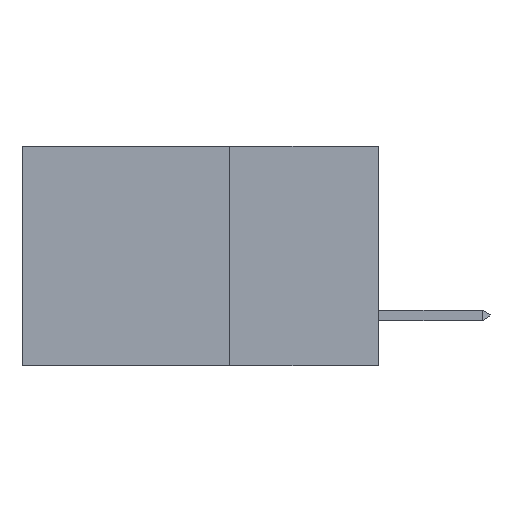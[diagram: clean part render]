
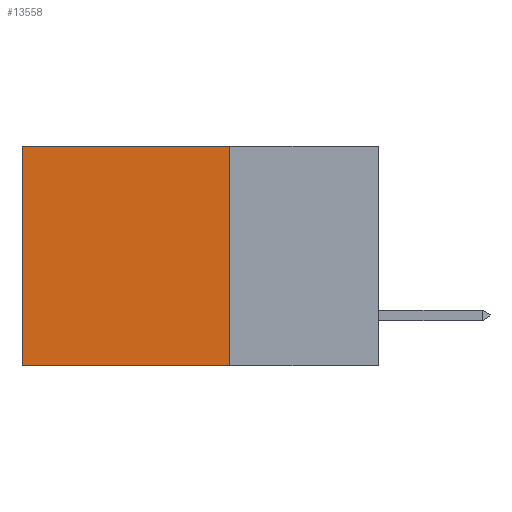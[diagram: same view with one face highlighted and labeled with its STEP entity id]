
A CAD part, left-side view. The second image highlights one B-rep face of the part: STEP entity #13558.
In plain terms, the highlighted planar face has unit normal (-1, 0, 0).
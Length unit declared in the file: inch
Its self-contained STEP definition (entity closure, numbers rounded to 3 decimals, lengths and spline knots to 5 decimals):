
#836 = ORIENTED_EDGE ( 'NONE', *, *, #20649, .T. ) ;
#1356 = CARTESIAN_POINT ( 'NONE',  ( 0.2615, 0.6, -0.37 ) ) ;
#1430 = EDGE_LOOP ( 'NONE', ( #836, #12405, #22193, #13598 ) ) ;
#1436 = DIRECTION ( 'NONE',  ( 0., 0., -1. ) ) ;
#1724 = CARTESIAN_POINT ( 'NONE',  ( 0.2615, 0.6, 0. ) ) ;
#2006 = EDGE_CURVE ( 'NONE', #5939, #5750, #13327, .T. ) ;
#3229 = DIRECTION ( 'NONE',  ( 0., 1., 0. ) ) ;
#4410 = LINE ( 'NONE', #1356, #17675 ) ;
#4940 = PLANE ( 'NONE',  #7764 ) ;
#5454 = VERTEX_POINT ( 'NONE', #18289 ) ;
#5750 = VERTEX_POINT ( 'NONE', #1724 ) ;
#5939 = VERTEX_POINT ( 'NONE', #19755 ) ;
#7031 = DIRECTION ( 'NONE',  ( 0., 1., 0. ) ) ;
#7764 = AXIS2_PLACEMENT_3D ( 'NONE', #10252, #17168, #1436 ) ;
#8415 = VECTOR ( 'NONE', #3229, 39.37008 ) ;
#8834 = CARTESIAN_POINT ( 'NONE',  ( 0.2615, 0.25, -0.37 ) ) ;
#9804 = FACE_OUTER_BOUND ( 'NONE', #1430, .T. ) ;
#10252 = CARTESIAN_POINT ( 'NONE',  ( 0.2615, 0.25, -0.37 ) ) ;
#10390 = CARTESIAN_POINT ( 'NONE',  ( 0.2615, 0.25, -0.37 ) ) ;
#12015 = LINE ( 'NONE', #8834, #19119 ) ;
#12405 = ORIENTED_EDGE ( 'NONE', *, *, #17701, .F. ) ;
#12940 = VECTOR ( 'NONE', #15413, 39.37008 ) ;
#13327 = LINE ( 'NONE', #13545, #8415 ) ;
#13545 = CARTESIAN_POINT ( 'NONE',  ( 0.2615, 0.25, 0. ) ) ;
#13558 = ADVANCED_FACE ( 'NONE', ( #9804 ), #4940, .F. ) ;
#13598 = ORIENTED_EDGE ( 'NONE', *, *, #2006, .T. ) ;
#13700 = LINE ( 'NONE', #10390, #12940 ) ;
#15413 = DIRECTION ( 'NONE',  ( 0., 0., -1. ) ) ;
#15892 = CARTESIAN_POINT ( 'NONE',  ( 0.2615, 0.25, -0.37 ) ) ;
#17168 = DIRECTION ( 'NONE',  ( 1., 0., 0. ) ) ;
#17675 = VECTOR ( 'NONE', #19850, 39.37008 ) ;
#17701 = EDGE_CURVE ( 'NONE', #21340, #5454, #12015, .T. ) ;
#18050 = EDGE_CURVE ( 'NONE', #5939, #21340, #13700, .T. ) ;
#18289 = CARTESIAN_POINT ( 'NONE',  ( 0.2615, 0.6, -0.37 ) ) ;
#19119 = VECTOR ( 'NONE', #7031, 39.37008 ) ;
#19755 = CARTESIAN_POINT ( 'NONE',  ( 0.2615, 0.25, 0. ) ) ;
#19850 = DIRECTION ( 'NONE',  ( 0., 0., -1. ) ) ;
#20649 = EDGE_CURVE ( 'NONE', #5750, #5454, #4410, .T. ) ;
#21340 = VERTEX_POINT ( 'NONE', #15892 ) ;
#22193 = ORIENTED_EDGE ( 'NONE', *, *, #18050, .F. ) ;
